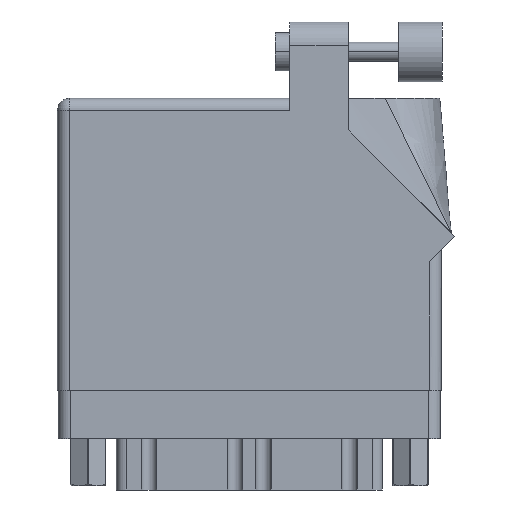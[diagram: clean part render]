
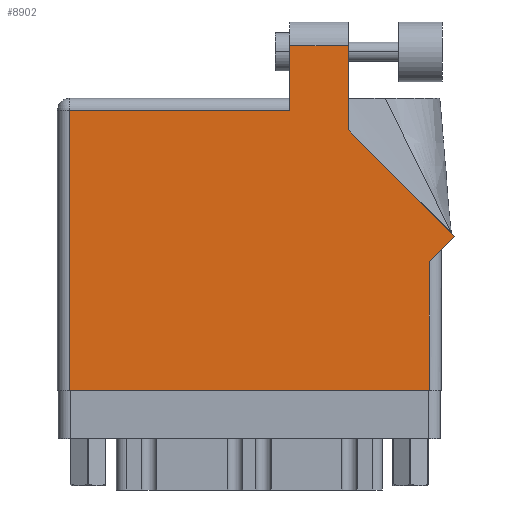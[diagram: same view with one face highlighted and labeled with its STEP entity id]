
A CAD part, front view. The second image highlights one B-rep face of the part: STEP entity #8902.
In plain terms, the highlighted face is planar.
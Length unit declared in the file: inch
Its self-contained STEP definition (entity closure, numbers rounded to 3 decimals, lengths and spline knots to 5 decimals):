
#79 = DIRECTION ( 'NONE',  ( -1., 0., 0. ) ) ;
#345 = LINE ( 'NONE', #39940, #31174 ) ;
#429 = CARTESIAN_POINT ( 'NONE',  ( 1.524, 1.36442, 0. ) ) ;
#936 = CARTESIAN_POINT ( 'NONE',  ( 1.217, 1.805, 0. ) ) ;
#1075 = ORIENTED_EDGE ( 'NONE', *, *, #20002, .T. ) ;
#1114 = LINE ( 'NONE', #23611, #17086 ) ;
#1400 = DIRECTION ( 'NONE',  ( 0.707, 0.707, 0. ) ) ;
#2140 = VECTOR ( 'NONE', #46713, 39.37008 ) ;
#2640 = ORIENTED_EDGE ( 'NONE', *, *, #4291, .T. ) ;
#2795 = CARTESIAN_POINT ( 'NONE',  ( 0., 1.468, 0. ) ) ;
#3152 = VERTEX_POINT ( 'NONE', #33774 ) ;
#3523 = DIRECTION ( 'NONE',  ( 0., 1., 0. ) ) ;
#3840 = CARTESIAN_POINT ( 'NONE',  ( 1.948, 0.675, 0. ) ) ;
#4291 = EDGE_CURVE ( 'NONE', #35551, #28473, #18654, .T. ) ;
#5240 = ORIENTED_EDGE ( 'NONE', *, *, #12187, .T. ) ;
#5647 = ORIENTED_EDGE ( 'NONE', *, *, #10609, .T. ) ;
#7345 = ORIENTED_EDGE ( 'NONE', *, *, #20981, .T. ) ;
#7582 = LINE ( 'NONE', #40232, #10877 ) ;
#8171 = EDGE_LOOP ( 'NONE', ( #7345, #5240, #35729, #1075, #5647, #2640, #23034, #8819, #28383 ) ) ;
#8819 = ORIENTED_EDGE ( 'NONE', *, *, #10080, .T. ) ;
#8902 = ADVANCED_FACE ( 'NONE', ( #22133 ), #44680, .F. ) ;
#10080 = EDGE_CURVE ( 'NONE', #26930, #45904, #19629, .T. ) ;
#10609 = EDGE_CURVE ( 'NONE', #3152, #35551, #1114, .T. ) ;
#10877 = VECTOR ( 'NONE', #3523, 39.37008 ) ;
#11680 = CARTESIAN_POINT ( 'NONE',  ( 0., 0., 0. ) ) ;
#11825 = VERTEX_POINT ( 'NONE', #936 ) ;
#12187 = EDGE_CURVE ( 'NONE', #31309, #11825, #345, .T. ) ;
#14586 = CARTESIAN_POINT ( 'NONE',  ( 1.524, 1.36442, 0. ) ) ;
#14666 = VERTEX_POINT ( 'NONE', #429 ) ;
#16656 = EDGE_CURVE ( 'NONE', #28473, #26930, #7582, .T. ) ;
#17086 = VECTOR ( 'NONE', #38043, 39.37008 ) ;
#18174 = DIRECTION ( 'NONE',  ( 1., 0., 0. ) ) ;
#18436 = DIRECTION ( 'NONE',  ( 0., 1., 0. ) ) ;
#18654 = LINE ( 'NONE', #11680, #30851 ) ;
#18862 = CARTESIAN_POINT ( 'NONE',  ( 2.08071, 0.80771, 0. ) ) ;
#19206 = VERTEX_POINT ( 'NONE', #26358 ) ;
#19389 = CARTESIAN_POINT ( 'NONE',  ( 2.01, 0.737, 0. ) ) ;
#19629 = LINE ( 'NONE', #19389, #29866 ) ;
#19665 = CARTESIAN_POINT ( 'NONE',  ( 1.524, 1.805, 0. ) ) ;
#20002 = EDGE_CURVE ( 'NONE', #19206, #3152, #28910, .T. ) ;
#20981 = EDGE_CURVE ( 'NONE', #14666, #31309, #25847, .T. ) ;
#22133 = FACE_OUTER_BOUND ( 'NONE', #8171, .T. ) ;
#22755 = EDGE_CURVE ( 'NONE', #11825, #19206, #39775, .T. ) ;
#23034 = ORIENTED_EDGE ( 'NONE', *, *, #16656, .T. ) ;
#23611 = CARTESIAN_POINT ( 'NONE',  ( 0.062, 0., 0. ) ) ;
#23659 = VECTOR ( 'NONE', #18436, 39.37008 ) ;
#24764 = EDGE_CURVE ( 'NONE', #45904, #14666, #47237, .T. ) ;
#25847 = LINE ( 'NONE', #14586, #23659 ) ;
#26358 = CARTESIAN_POINT ( 'NONE',  ( 1.217, 1.468, 0. ) ) ;
#26415 = DIRECTION ( 'NONE',  ( 0., 0., -1. ) ) ;
#26930 = VERTEX_POINT ( 'NONE', #3840 ) ;
#28383 = ORIENTED_EDGE ( 'NONE', *, *, #24764, .T. ) ;
#28473 = VERTEX_POINT ( 'NONE', #34178 ) ;
#28910 = LINE ( 'NONE', #2795, #2140 ) ;
#29822 = DIRECTION ( 'NONE',  ( -1., 0., 0. ) ) ;
#29866 = VECTOR ( 'NONE', #1400, 39.37008 ) ;
#30851 = VECTOR ( 'NONE', #18174, 39.37008 ) ;
#31174 = VECTOR ( 'NONE', #29822, 39.37008 ) ;
#31309 = VERTEX_POINT ( 'NONE', #19665 ) ;
#33774 = CARTESIAN_POINT ( 'NONE',  ( 0.062, 1.468, 0. ) ) ;
#34178 = CARTESIAN_POINT ( 'NONE',  ( 1.948, 0., 0. ) ) ;
#35551 = VERTEX_POINT ( 'NONE', #45698 ) ;
#35729 = ORIENTED_EDGE ( 'NONE', *, *, #22755, .T. ) ;
#36428 = CARTESIAN_POINT ( 'NONE',  ( 2.08071, 0.80771, 0. ) ) ;
#36946 = VECTOR ( 'NONE', #43149, 39.37008 ) ;
#36948 = AXIS2_PLACEMENT_3D ( 'NONE', #40606, #26415, #79 ) ;
#38043 = DIRECTION ( 'NONE',  ( 0., -1., 0. ) ) ;
#38822 = CARTESIAN_POINT ( 'NONE',  ( 1.217, 1.53, 0. ) ) ;
#39549 = DIRECTION ( 'NONE',  ( -0.707, 0.707, 0. ) ) ;
#39775 = LINE ( 'NONE', #38822, #36946 ) ;
#39940 = CARTESIAN_POINT ( 'NONE',  ( 1.217, 1.805, 0. ) ) ;
#40232 = CARTESIAN_POINT ( 'NONE',  ( 1.948, 0.737, 0. ) ) ;
#40606 = CARTESIAN_POINT ( 'NONE',  ( 0., 1.53, 0. ) ) ;
#43149 = DIRECTION ( 'NONE',  ( 0., -1., 0. ) ) ;
#44680 = PLANE ( 'NONE',  #36948 ) ;
#44737 = VECTOR ( 'NONE', #39549, 39.37008 ) ;
#45698 = CARTESIAN_POINT ( 'NONE',  ( 0.062, 0., 0. ) ) ;
#45904 = VERTEX_POINT ( 'NONE', #18862 ) ;
#46713 = DIRECTION ( 'NONE',  ( -1., 0., 0. ) ) ;
#47237 = LINE ( 'NONE', #36428, #44737 ) ;
